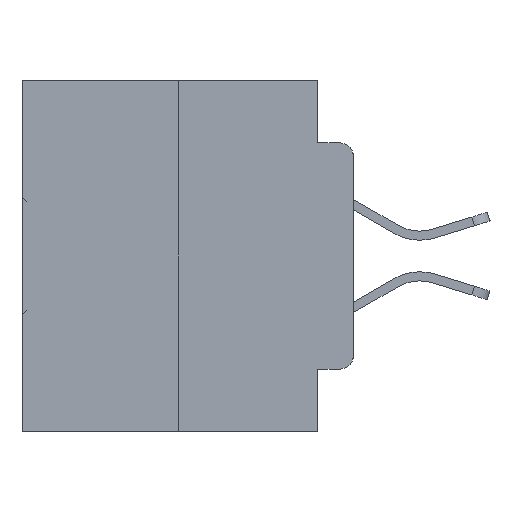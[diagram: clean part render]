
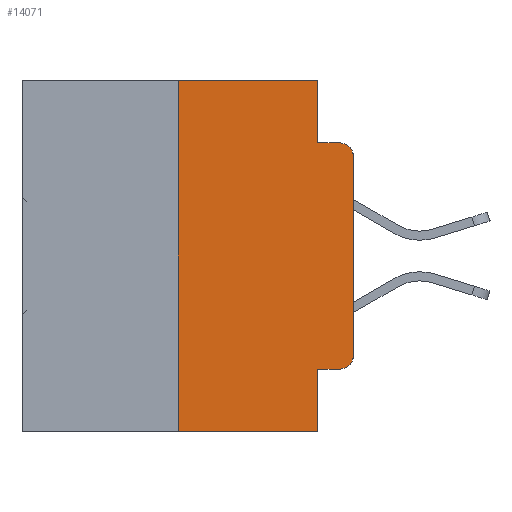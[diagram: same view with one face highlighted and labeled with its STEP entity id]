
A CAD part, left-side view. The second image highlights one B-rep face of the part: STEP entity #14071.
In plain terms, the highlighted planar face has unit normal (-1, 0, 0).
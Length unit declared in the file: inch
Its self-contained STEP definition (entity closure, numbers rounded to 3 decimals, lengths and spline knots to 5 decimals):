
#221 = DIRECTION ( 'NONE',  ( -1., 0., 0. ) ) ;
#481 = CARTESIAN_POINT ( 'NONE',  ( 0., 0.02, -0.0885 ) ) ;
#916 = EDGE_CURVE ( 'NONE', #24915, #1592, #18393, .T. ) ;
#1592 = VERTEX_POINT ( 'NONE', #481 ) ;
#1846 = CARTESIAN_POINT ( 'NONE',  ( 0., 0.25, 0. ) ) ;
#1857 = VERTEX_POINT ( 'NONE', #14186 ) ;
#2071 = CARTESIAN_POINT ( 'NONE',  ( 0., 0.051, 0. ) ) ;
#2377 = CARTESIAN_POINT ( 'NONE',  ( 0., 0.473, 0. ) ) ;
#2952 = CARTESIAN_POINT ( 'NONE',  ( 0., 0.051, -0.5 ) ) ;
#3121 = DIRECTION ( 'NONE',  ( 1., 0., 0. ) ) ;
#3168 = ORIENTED_EDGE ( 'NONE', *, *, #5668, .F. ) ;
#3747 = DIRECTION ( 'NONE',  ( 0., -1., 0. ) ) ;
#4205 = VERTEX_POINT ( 'NONE', #1846 ) ;
#5058 = DIRECTION ( 'NONE',  ( 0., -1., 0. ) ) ;
#5081 = CARTESIAN_POINT ( 'NONE',  ( 0., 0.051, -0.0885 ) ) ;
#5668 = EDGE_CURVE ( 'NONE', #23975, #9901, #26218, .T. ) ;
#5676 = VERTEX_POINT ( 'NONE', #5081 ) ;
#5697 = VECTOR ( 'NONE', #28867, 39.37008 ) ;
#7071 = ORIENTED_EDGE ( 'NONE', *, *, #19215, .F. ) ;
#7328 = VERTEX_POINT ( 'NONE', #22347 ) ;
#7542 = AXIS2_PLACEMENT_3D ( 'NONE', #8791, #3121, #19567 ) ;
#7588 = LINE ( 'NONE', #23958, #33836 ) ;
#7593 = ORIENTED_EDGE ( 'NONE', *, *, #34345, .T. ) ;
#7696 = EDGE_CURVE ( 'NONE', #5676, #1592, #30035, .T. ) ;
#7719 = LINE ( 'NONE', #15312, #5697 ) ;
#7904 = ORIENTED_EDGE ( 'NONE', *, *, #23864, .T. ) ;
#8177 = AXIS2_PLACEMENT_3D ( 'NONE', #23941, #13732, #18850 ) ;
#8791 = CARTESIAN_POINT ( 'NONE',  ( 0., 0.473, 0. ) ) ;
#8888 = VECTOR ( 'NONE', #29247, 39.37008 ) ;
#9038 = VECTOR ( 'NONE', #3747, 39.37008 ) ;
#9293 = VECTOR ( 'NONE', #5058, 39.37008 ) ;
#9877 = ORIENTED_EDGE ( 'NONE', *, *, #13142, .F. ) ;
#9901 = VERTEX_POINT ( 'NONE', #2952 ) ;
#10052 = ORIENTED_EDGE ( 'NONE', *, *, #7696, .F. ) ;
#10663 = LINE ( 'NONE', #32170, #26426 ) ;
#10994 = DIRECTION ( 'NONE',  ( 0., 0., -1. ) ) ;
#11023 = CARTESIAN_POINT ( 'NONE',  ( 0., 0., -0.1085 ) ) ;
#11438 = PLANE ( 'NONE',  #7542 ) ;
#11520 = CARTESIAN_POINT ( 'NONE',  ( 0., 0.25, 0. ) ) ;
#12084 = CIRCLE ( 'NONE', #8177, 0.02 ) ;
#12244 = VECTOR ( 'NONE', #23888, 39.37008 ) ;
#12704 = ORIENTED_EDGE ( 'NONE', *, *, #22925, .F. ) ;
#13142 = EDGE_CURVE ( 'NONE', #7328, #4205, #19464, .T. ) ;
#13638 = CARTESIAN_POINT ( 'NONE',  ( 0., 0.02, -0.1085 ) ) ;
#13677 = CARTESIAN_POINT ( 'NONE',  ( 0., 0.02, -0.4115 ) ) ;
#13732 = DIRECTION ( 'NONE',  ( -1., 0., 0. ) ) ;
#14071 = ADVANCED_FACE ( 'NONE', ( #27273 ), #11438, .F. ) ;
#14186 = CARTESIAN_POINT ( 'NONE',  ( 0., 0., -0.3915 ) ) ;
#15312 = CARTESIAN_POINT ( 'NONE',  ( 0., 0.051, 0. ) ) ;
#17848 = CARTESIAN_POINT ( 'NONE',  ( 0., 0.051, 0. ) ) ;
#18337 = DIRECTION ( 'NONE',  ( 0., 0., 1. ) ) ;
#18393 = CIRCLE ( 'NONE', #33055, 0.02 ) ;
#18418 = ORIENTED_EDGE ( 'NONE', *, *, #916, .T. ) ;
#18466 = LINE ( 'NONE', #29223, #9293 ) ;
#18850 = DIRECTION ( 'NONE',  ( 0., 0., -1. ) ) ;
#19007 = ORIENTED_EDGE ( 'NONE', *, *, #30044, .T. ) ;
#19215 = EDGE_CURVE ( 'NONE', #4205, #28884, #26536, .T. ) ;
#19229 = VERTEX_POINT ( 'NONE', #13677 ) ;
#19464 = LINE ( 'NONE', #11520, #20453 ) ;
#19567 = DIRECTION ( 'NONE',  ( 0., 0., -1. ) ) ;
#20453 = VECTOR ( 'NONE', #24551, 39.37008 ) ;
#21420 = DIRECTION ( 'NONE',  ( 0., -1., 0. ) ) ;
#22123 = CARTESIAN_POINT ( 'NONE',  ( 0., 0.051, -0.0885 ) ) ;
#22347 = CARTESIAN_POINT ( 'NONE',  ( 0., 0.25, -0.5 ) ) ;
#22925 = EDGE_CURVE ( 'NONE', #28884, #5676, #7719, .T. ) ;
#23864 = EDGE_CURVE ( 'NONE', #1857, #24915, #7588, .T. ) ;
#23888 = DIRECTION ( 'NONE',  ( 0., -1., 0. ) ) ;
#23941 = CARTESIAN_POINT ( 'NONE',  ( 0., 0.02, -0.3915 ) ) ;
#23958 = CARTESIAN_POINT ( 'NONE',  ( 0., 0., 0. ) ) ;
#23975 = VERTEX_POINT ( 'NONE', #30138 ) ;
#24551 = DIRECTION ( 'NONE',  ( 0., 0., 1. ) ) ;
#24915 = VERTEX_POINT ( 'NONE', #11023 ) ;
#26218 = LINE ( 'NONE', #2071, #8888 ) ;
#26426 = VECTOR ( 'NONE', #21420, 39.37008 ) ;
#26536 = LINE ( 'NONE', #2377, #12244 ) ;
#26682 = EDGE_LOOP ( 'NONE', ( #7904, #18418, #10052, #12704, #7071, #9877, #19007, #3168, #7593, #32333 ) ) ;
#27273 = FACE_OUTER_BOUND ( 'NONE', #26682, .T. ) ;
#28867 = DIRECTION ( 'NONE',  ( 0., 0., -1. ) ) ;
#28884 = VERTEX_POINT ( 'NONE', #17848 ) ;
#29223 = CARTESIAN_POINT ( 'NONE',  ( 0., 0.473, -0.5 ) ) ;
#29247 = DIRECTION ( 'NONE',  ( 0., 0., -1. ) ) ;
#29558 = EDGE_CURVE ( 'NONE', #19229, #1857, #12084, .T. ) ;
#30035 = LINE ( 'NONE', #22123, #9038 ) ;
#30044 = EDGE_CURVE ( 'NONE', #7328, #9901, #18466, .T. ) ;
#30138 = CARTESIAN_POINT ( 'NONE',  ( 0., 0.051, -0.4115 ) ) ;
#32170 = CARTESIAN_POINT ( 'NONE',  ( 0., 0.051, -0.4115 ) ) ;
#32333 = ORIENTED_EDGE ( 'NONE', *, *, #29558, .T. ) ;
#33055 = AXIS2_PLACEMENT_3D ( 'NONE', #13638, #221, #10994 ) ;
#33836 = VECTOR ( 'NONE', #18337, 39.37008 ) ;
#34345 = EDGE_CURVE ( 'NONE', #23975, #19229, #10663, .T. ) ;
